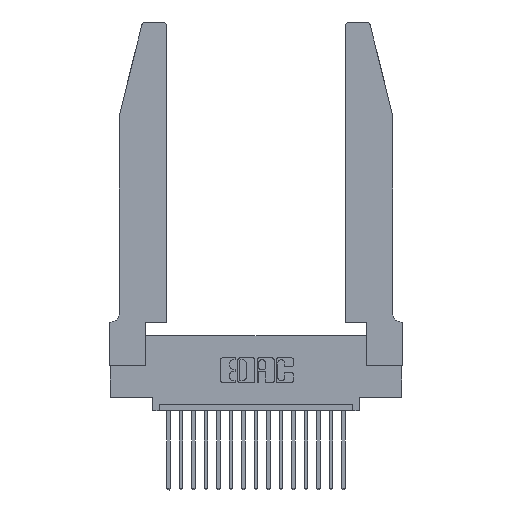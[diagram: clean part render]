
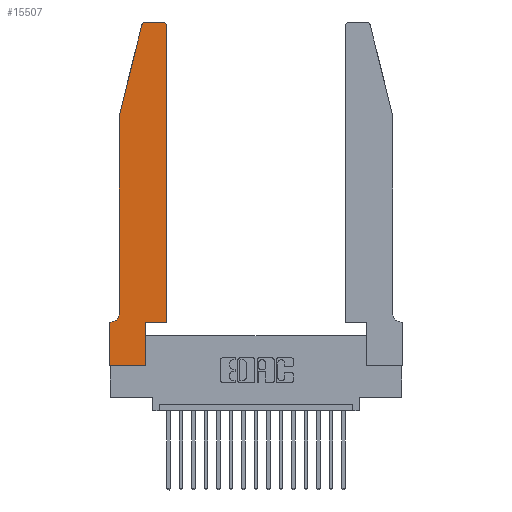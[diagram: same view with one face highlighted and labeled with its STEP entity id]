
A CAD part, top view. The second image highlights one B-rep face of the part: STEP entity #15507.
In plain terms, the highlighted planar face has unit normal (0, 0, 1).
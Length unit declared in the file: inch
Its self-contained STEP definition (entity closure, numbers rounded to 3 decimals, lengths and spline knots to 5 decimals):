
#19 = DIRECTION ( 'NONE',  ( 1., 0., 0. ) ) ;
#20 = EDGE_CURVE ( 'NONE', #10838, #12960, #9122, .T. ) ;
#324 = VERTEX_POINT ( 'NONE', #5366 ) ;
#747 = VERTEX_POINT ( 'NONE', #13356 ) ;
#1443 = CIRCLE ( 'NONE', #10432, 0.07 ) ;
#1658 = VECTOR ( 'NONE', #19, 39.37008 ) ;
#1659 = CARTESIAN_POINT ( 'NONE',  ( 0.2865, 0.35, 0.37 ) ) ;
#1753 = EDGE_CURVE ( 'NONE', #3949, #7617, #19315, .T. ) ;
#1849 = DIRECTION ( 'NONE',  ( -1., 0., 0. ) ) ;
#2143 = CARTESIAN_POINT ( 'NONE',  ( 0.0755, 0.42, 0.37 ) ) ;
#2311 = DIRECTION ( 'NONE',  ( -1., 0., 0. ) ) ;
#2808 = DIRECTION ( 'NONE',  ( 1., 0., 0. ) ) ;
#3066 = DIRECTION ( 'NONE',  ( 0., 0., 1. ) ) ;
#3076 = CARTESIAN_POINT ( 'NONE',  ( 0.4505, 0.35, 0.37 ) ) ;
#3116 = CARTESIAN_POINT ( 'NONE',  ( 0.2865, 0., 0.37 ) ) ;
#3299 = ORIENTED_EDGE ( 'NONE', *, *, #8998, .T. ) ;
#3400 = VECTOR ( 'NONE', #18568, 39.37008 ) ;
#3422 = AXIS2_PLACEMENT_3D ( 'NONE', #7229, #11966, #2808 ) ;
#3757 = VERTEX_POINT ( 'NONE', #7741 ) ;
#3820 = CIRCLE ( 'NONE', #3422, 0.03 ) ;
#3866 = CARTESIAN_POINT ( 'NONE',  ( 0.0755, 2., 0.37 ) ) ;
#3949 = VERTEX_POINT ( 'NONE', #5046 ) ;
#4206 = CARTESIAN_POINT ( 'NONE',  ( 0., 0., 0.37 ) ) ;
#4268 = EDGE_CURVE ( 'NONE', #13485, #16897, #17945, .T. ) ;
#4318 = CARTESIAN_POINT ( 'NONE',  ( 0., 0.35, 0.37 ) ) ;
#4328 = EDGE_CURVE ( 'NONE', #15072, #13485, #7170, .T. ) ;
#4997 = DIRECTION ( 'NONE',  ( 0., -1., 0. ) ) ;
#5046 = CARTESIAN_POINT ( 'NONE',  ( 0.0755, 2., 0.37 ) ) ;
#5366 = CARTESIAN_POINT ( 'NONE',  ( 0., 0., 0.37 ) ) ;
#5564 = EDGE_CURVE ( 'NONE', #324, #15072, #6673, .T. ) ;
#5653 = CARTESIAN_POINT ( 'NONE',  ( 0.2865, 0.35, 0.37 ) ) ;
#5655 = AXIS2_PLACEMENT_3D ( 'NONE', #18515, #12537, #14094 ) ;
#5824 = ORIENTED_EDGE ( 'NONE', *, *, #10453, .T. ) ;
#5889 = VERTEX_POINT ( 'NONE', #19461 ) ;
#6288 = PLANE ( 'NONE',  #5655 ) ;
#6556 = CARTESIAN_POINT ( 'NONE',  ( 0.0755, 0.35, 0.37 ) ) ;
#6673 = LINE ( 'NONE', #4206, #10929 ) ;
#6724 = ORIENTED_EDGE ( 'NONE', *, *, #4328, .T. ) ;
#6746 = VECTOR ( 'NONE', #1849, 39.37008 ) ;
#7170 = LINE ( 'NONE', #1659, #13638 ) ;
#7229 = CARTESIAN_POINT ( 'NONE',  ( 0.284, 2.72, 0.37 ) ) ;
#7486 = CARTESIAN_POINT ( 'NONE',  ( 0.4205, 2.72, 0.37 ) ) ;
#7495 = VERTEX_POINT ( 'NONE', #9772 ) ;
#7617 = VERTEX_POINT ( 'NONE', #2143 ) ;
#7741 = CARTESIAN_POINT ( 'NONE',  ( 0.25487, 2.72718, 0.37 ) ) ;
#8011 = CARTESIAN_POINT ( 'NONE',  ( 0., 0., 0.37 ) ) ;
#8183 = LINE ( 'NONE', #8011, #3400 ) ;
#8998 = EDGE_CURVE ( 'NONE', #12960, #324, #8183, .T. ) ;
#9059 = DIRECTION ( 'NONE',  ( -1., 0., 0. ) ) ;
#9073 = DIRECTION ( 'NONE',  ( 1., 0., 0. ) ) ;
#9122 = LINE ( 'NONE', #6556, #6746 ) ;
#9260 = ORIENTED_EDGE ( 'NONE', *, *, #11712, .T. ) ;
#9732 = CIRCLE ( 'NONE', #14535, 0.03 ) ;
#9772 = CARTESIAN_POINT ( 'NONE',  ( 0.4205, 2.75, 0.37 ) ) ;
#10353 = ORIENTED_EDGE ( 'NONE', *, *, #19560, .T. ) ;
#10432 = AXIS2_PLACEMENT_3D ( 'NONE', #18973, #11466, #2311 ) ;
#10453 = EDGE_CURVE ( 'NONE', #7617, #10838, #1443, .T. ) ;
#10838 = VERTEX_POINT ( 'NONE', #15472 ) ;
#10929 = VECTOR ( 'NONE', #11542, 39.37008 ) ;
#11009 = DIRECTION ( 'NONE',  ( 0., 1., 0. ) ) ;
#11253 = CARTESIAN_POINT ( 'NONE',  ( 0.4505, 0.35, 0.37 ) ) ;
#11466 = DIRECTION ( 'NONE',  ( 0., 0., -1. ) ) ;
#11542 = DIRECTION ( 'NONE',  ( 1., 0., 0. ) ) ;
#11712 = EDGE_CURVE ( 'NONE', #747, #3757, #3820, .T. ) ;
#11966 = DIRECTION ( 'NONE',  ( 0., 0., 1. ) ) ;
#12536 = ORIENTED_EDGE ( 'NONE', *, *, #20, .T. ) ;
#12537 = DIRECTION ( 'NONE',  ( 0., 0., 1. ) ) ;
#12569 = ORIENTED_EDGE ( 'NONE', *, *, #5564, .T. ) ;
#12793 = CARTESIAN_POINT ( 'NONE',  ( 0.0755, 2., 0.37 ) ) ;
#12895 = EDGE_CURVE ( 'NONE', #16897, #5889, #18097, .T. ) ;
#12960 = VERTEX_POINT ( 'NONE', #4318 ) ;
#13212 = EDGE_CURVE ( 'NONE', #3757, #3949, #18566, .T. ) ;
#13311 = ORIENTED_EDGE ( 'NONE', *, *, #1753, .T. ) ;
#13356 = CARTESIAN_POINT ( 'NONE',  ( 0.284, 2.75, 0.37 ) ) ;
#13450 = ORIENTED_EDGE ( 'NONE', *, *, #4268, .T. ) ;
#13485 = VERTEX_POINT ( 'NONE', #5653 ) ;
#13638 = VECTOR ( 'NONE', #11009, 39.37008 ) ;
#13960 = ORIENTED_EDGE ( 'NONE', *, *, #17256, .T. ) ;
#14094 = DIRECTION ( 'NONE',  ( 1., 0., 0. ) ) ;
#14535 = AXIS2_PLACEMENT_3D ( 'NONE', #7486, #3066, #9073 ) ;
#15072 = VERTEX_POINT ( 'NONE', #3116 ) ;
#15233 = VECTOR ( 'NONE', #19152, 39.37008 ) ;
#15472 = CARTESIAN_POINT ( 'NONE',  ( 0.0055, 0.35, 0.37 ) ) ;
#15507 = ADVANCED_FACE ( 'NONE', ( #19432 ), #6288, .T. ) ;
#15694 = ORIENTED_EDGE ( 'NONE', *, *, #13212, .T. ) ;
#16267 = LINE ( 'NONE', #16766, #18673 ) ;
#16523 = ORIENTED_EDGE ( 'NONE', *, *, #12895, .T. ) ;
#16766 = CARTESIAN_POINT ( 'NONE',  ( 0.2605, 2.75, 0.37 ) ) ;
#16897 = VERTEX_POINT ( 'NONE', #3076 ) ;
#17256 = EDGE_CURVE ( 'NONE', #7495, #747, #16267, .T. ) ;
#17291 = DIRECTION ( 'NONE',  ( 0., 1., 0. ) ) ;
#17411 = VECTOR ( 'NONE', #4997, 39.37008 ) ;
#17869 = VECTOR ( 'NONE', #17291, 39.37008 ) ;
#17945 = LINE ( 'NONE', #19701, #1658 ) ;
#18097 = LINE ( 'NONE', #11253, #17869 ) ;
#18515 = CARTESIAN_POINT ( 'NONE',  ( 0., 0.35, 0.37 ) ) ;
#18566 = LINE ( 'NONE', #3866, #15233 ) ;
#18568 = DIRECTION ( 'NONE',  ( 0., -1., 0. ) ) ;
#18673 = VECTOR ( 'NONE', #9059, 39.37008 ) ;
#18769 = EDGE_LOOP ( 'NONE', ( #13960, #9260, #15694, #13311, #5824, #12536, #3299, #12569, #6724, #13450, #16523, #10353 ) ) ;
#18973 = CARTESIAN_POINT ( 'NONE',  ( 0.0055, 0.42, 0.37 ) ) ;
#19152 = DIRECTION ( 'NONE',  ( -0.239, -0.971, 0. ) ) ;
#19315 = LINE ( 'NONE', #12793, #17411 ) ;
#19432 = FACE_OUTER_BOUND ( 'NONE', #18769, .T. ) ;
#19461 = CARTESIAN_POINT ( 'NONE',  ( 0.4505, 2.72, 0.37 ) ) ;
#19560 = EDGE_CURVE ( 'NONE', #5889, #7495, #9732, .T. ) ;
#19701 = CARTESIAN_POINT ( 'NONE',  ( 0.4505, 0.35, 0.37 ) ) ;
